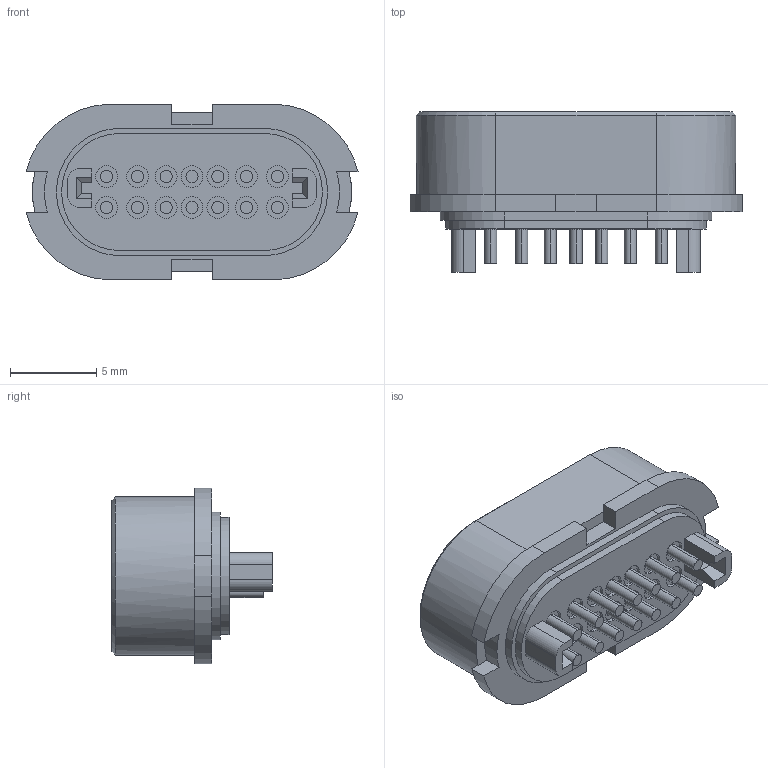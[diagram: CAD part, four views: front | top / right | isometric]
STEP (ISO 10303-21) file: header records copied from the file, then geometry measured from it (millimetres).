
FILE_DESCRIPTION (( 'STEP AP214' ), '1' );
FILE_NAME ('685A14C4220115E.STEP', '2023-05-01T18:24:43', ( '' ), ( '' ), 'SwSTEP 2.0', 'SolidWorks 2020', '' );
FILE_SCHEMA (( 'AUTOMOTIVE_DESIGN' ));
Length unit declared in the file: millimetre
Products named in the file (1): 685A14C4220115E
Bounding box: 19.28 x 9.3 x 10.2 mm (x, y, z)
Volume: 882.8 mm3; surface area: 876 mm2
Topology: 1 solids, 1 shells, 278 faces, 664 edges, 422 vertices
Faces by surface type: cylinder 136, plane 110, sphere 28, cone 4
Entity records: 10800 total; most frequent: DIRECTION 1474, CARTESIAN_POINT 1281, ORIENTED_EDGE 1216, EDGE_CURVE 608, AXIS2_PLACEMENT_3D 587, VERTEX_POINT 394, EDGE_LOOP 340, CIRCLE 308
